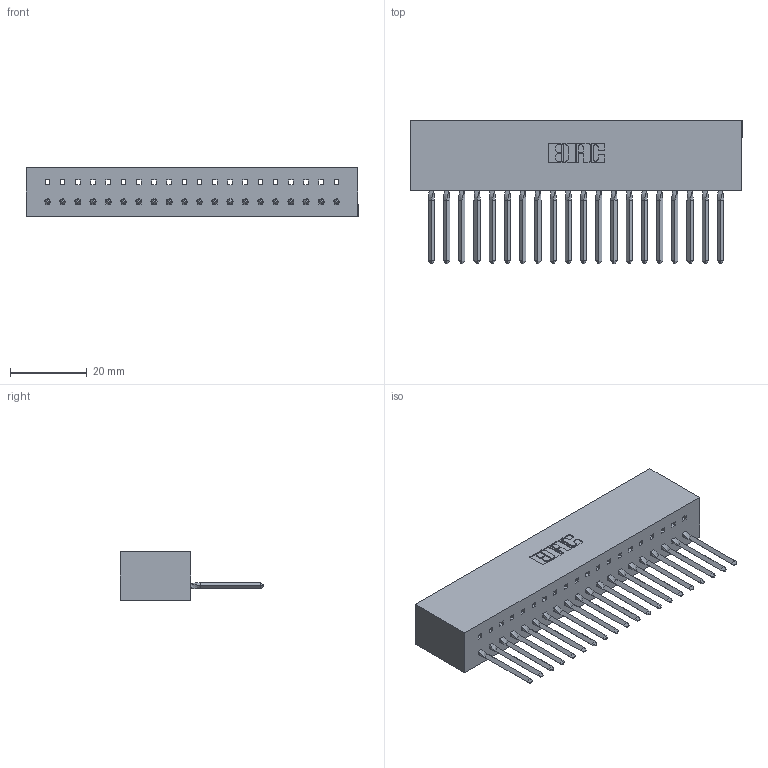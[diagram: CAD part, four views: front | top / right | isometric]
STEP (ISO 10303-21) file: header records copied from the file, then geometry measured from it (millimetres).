
FILE_DESCRIPTION (( 'STEP AP203' ), '1' );
FILE_NAME ('317-020-542-601.STEP', '2020-02-27T16:27:10', ( '' ), ( '' ), 'SwSTEP 2.0', 'SolidWorks 2016', '' );
FILE_SCHEMA (( 'CONFIG_CONTROL_DESIGN' ));
Length unit declared in the file: inch
Products named in the file (3): 317 Part_Lugless; 317-290-003_542; 317-020-542-601
Assembly tree (21 placements, depth 2):
  317-020-542-601
    317 Part_Lugless
    317-290-003_542  x20
Bounding box: 86.46 x 37.34 x 12.7 mm (x, y, z)
Volume: 14357.6 mm3; surface area: 17062.4 mm2
Topology: 21 solids, 21 shells, 1590 faces, 4579 edges, 2958 vertices
Faces by surface type: plane 1330, cylinder 180, bspline 80
Entity records: 29947 total; most frequent: CARTESIAN_POINT 5561, ORIENTED_EDGE 5244, DIRECTION 4402, EDGE_CURVE 2622, LINE 2460, VECTOR 2460, VERTEX_POINT 1742, AXIS2_PLACEMENT_3D 971
